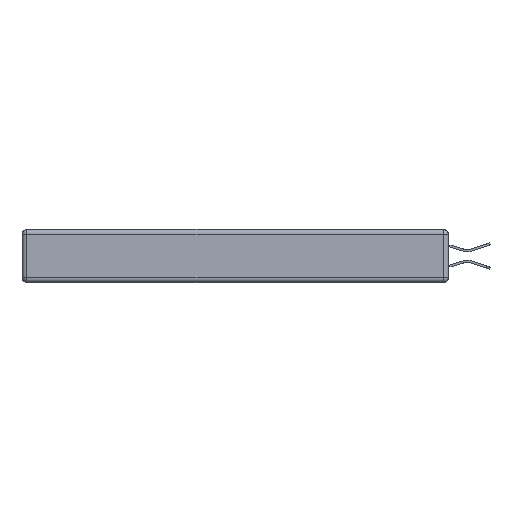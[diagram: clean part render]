
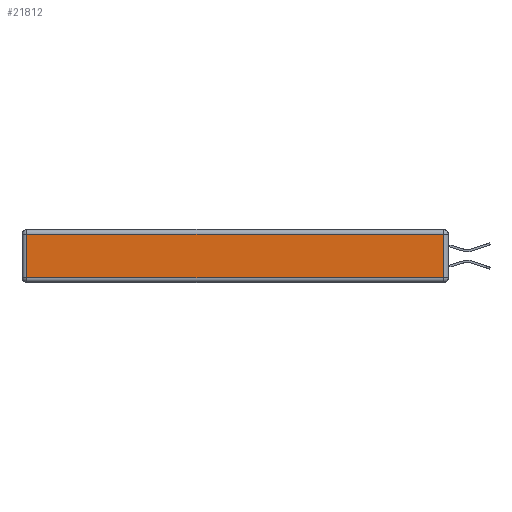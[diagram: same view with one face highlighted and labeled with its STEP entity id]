
A CAD part, left-side view. The second image highlights one B-rep face of the part: STEP entity #21812.
In plain terms, the highlighted planar face has unit normal (-1, 0, 0).
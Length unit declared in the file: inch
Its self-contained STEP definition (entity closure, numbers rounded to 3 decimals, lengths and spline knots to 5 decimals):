
#1024 = CARTESIAN_POINT ( 'NONE',  ( 0., 0.03, -0.313 ) ) ;
#1150 = EDGE_CURVE ( 'NONE', #13309, #26086, #28308, .T. ) ;
#1521 = VERTEX_POINT ( 'NONE', #1024 ) ;
#2540 = DIRECTION ( 'NONE',  ( 0., 0., -1. ) ) ;
#2668 = CARTESIAN_POINT ( 'NONE',  ( 0., 0., -0.343 ) ) ;
#4781 = FACE_OUTER_BOUND ( 'NONE', #6888, .T. ) ;
#5931 = CARTESIAN_POINT ( 'NONE',  ( 0., 2.75, -0.03 ) ) ;
#6888 = EDGE_LOOP ( 'NONE', ( #21983, #17266, #13040, #26629 ) ) ;
#7634 = EDGE_CURVE ( 'NONE', #26086, #22796, #24808, .T. ) ;
#8786 = EDGE_CURVE ( 'NONE', #1521, #13309, #10688, .T. ) ;
#9085 = AXIS2_PLACEMENT_3D ( 'NONE', #2668, #26380, #17088 ) ;
#10663 = VECTOR ( 'NONE', #27501, 39.37008 ) ;
#10688 = LINE ( 'NONE', #25358, #10663 ) ;
#11306 = DIRECTION ( 'NONE',  ( 0., 1., 0. ) ) ;
#12249 = VECTOR ( 'NONE', #2540, 39.37008 ) ;
#12549 = CARTESIAN_POINT ( 'NONE',  ( 0., 0.03, -0.03 ) ) ;
#12757 = CARTESIAN_POINT ( 'NONE',  ( 0., 0., -0.313 ) ) ;
#13040 = ORIENTED_EDGE ( 'NONE', *, *, #1150, .T. ) ;
#13309 = VERTEX_POINT ( 'NONE', #12549 ) ;
#17088 = DIRECTION ( 'NONE',  ( 0., 0., 1. ) ) ;
#17266 = ORIENTED_EDGE ( 'NONE', *, *, #8786, .T. ) ;
#19327 = VECTOR ( 'NONE', #29135, 39.37008 ) ;
#21812 = ADVANCED_FACE ( 'NONE', ( #4781 ), #28844, .T. ) ;
#21983 = ORIENTED_EDGE ( 'NONE', *, *, #23596, .T. ) ;
#22796 = VERTEX_POINT ( 'NONE', #30475 ) ;
#23596 = EDGE_CURVE ( 'NONE', #22796, #1521, #26431, .T. ) ;
#24808 = LINE ( 'NONE', #26454, #12249 ) ;
#25358 = CARTESIAN_POINT ( 'NONE',  ( 0., 0.03, -0.343 ) ) ;
#25760 = CARTESIAN_POINT ( 'NONE',  ( 0., 2.72, -0.03 ) ) ;
#26086 = VERTEX_POINT ( 'NONE', #25760 ) ;
#26100 = VECTOR ( 'NONE', #11306, 39.37008 ) ;
#26380 = DIRECTION ( 'NONE',  ( -1., 0., 0. ) ) ;
#26431 = LINE ( 'NONE', #12757, #19327 ) ;
#26454 = CARTESIAN_POINT ( 'NONE',  ( 0., 2.72, -0.343 ) ) ;
#26629 = ORIENTED_EDGE ( 'NONE', *, *, #7634, .T. ) ;
#27501 = DIRECTION ( 'NONE',  ( 0., 0., 1. ) ) ;
#28308 = LINE ( 'NONE', #5931, #26100 ) ;
#28844 = PLANE ( 'NONE',  #9085 ) ;
#29135 = DIRECTION ( 'NONE',  ( 0., -1., 0. ) ) ;
#30475 = CARTESIAN_POINT ( 'NONE',  ( 0., 2.72, -0.313 ) ) ;
